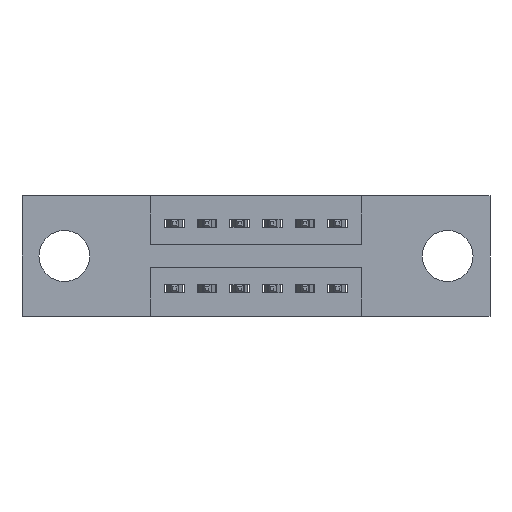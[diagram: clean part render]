
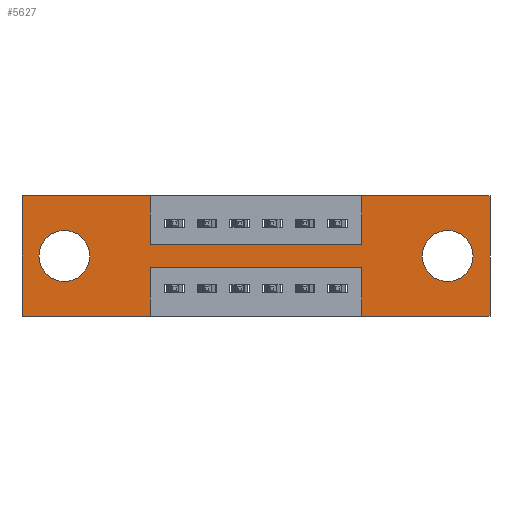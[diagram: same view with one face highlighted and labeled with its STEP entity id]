
A CAD part, front view. The second image highlights one B-rep face of the part: STEP entity #5627.
In plain terms, the highlighted planar face has unit normal (0, -1, 0).
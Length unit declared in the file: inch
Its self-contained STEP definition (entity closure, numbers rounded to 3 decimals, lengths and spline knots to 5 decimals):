
#52 = DIRECTION ( 'NONE',  ( 1., 0., 0. ) ) ;
#59 = DIRECTION ( 'NONE',  ( 0., 0., -1. ) ) ;
#96 = VERTEX_POINT ( 'NONE', #4070 ) ;
#128 = CARTESIAN_POINT ( 'NONE',  ( 0.3925, 0., -0.37 ) ) ;
#204 = DIRECTION ( 'NONE',  ( 0., 0., 1. ) ) ;
#215 = CARTESIAN_POINT ( 'NONE',  ( 0., 0., -0.37 ) ) ;
#245 = VERTEX_POINT ( 'NONE', #5455 ) ;
#251 = CARTESIAN_POINT ( 'NONE',  ( 0.13, 0., -0.263 ) ) ;
#255 = EDGE_CURVE ( 'NONE', #1596, #6113, #8047, .T. ) ;
#288 = VERTEX_POINT ( 'NONE', #5381 ) ;
#326 = DIRECTION ( 'NONE',  ( -1., 0., 0. ) ) ;
#418 = DIRECTION ( 'NONE',  ( 0., 0., -1. ) ) ;
#671 = VECTOR ( 'NONE', #3978, 39.37008 ) ;
#684 = VECTOR ( 'NONE', #4832, 39.37008 ) ;
#730 = EDGE_LOOP ( 'NONE', ( #4895, #5170, #6230, #2188, #3223, #6714, #6895, #7309, #1668, #2954, #6140, #4345 ) ) ;
#1065 = VECTOR ( 'NONE', #418, 39.37008 ) ;
#1235 = CARTESIAN_POINT ( 'NONE',  ( 1.0425, 0., -0.37 ) ) ;
#1316 = AXIS2_PLACEMENT_3D ( 'NONE', #3298, #4785, #3431 ) ;
#1321 = VECTOR ( 'NONE', #9518, 39.37008 ) ;
#1490 = LINE ( 'NONE', #128, #671 ) ;
#1502 = CIRCLE ( 'NONE', #3021, 0.078 ) ;
#1596 = VERTEX_POINT ( 'NONE', #9465 ) ;
#1601 = CARTESIAN_POINT ( 'NONE',  ( 0.13, 0., -0.185 ) ) ;
#1655 = EDGE_CURVE ( 'NONE', #3205, #96, #9492, .T. ) ;
#1668 = ORIENTED_EDGE ( 'NONE', *, *, #4088, .F. ) ;
#1682 = DIRECTION ( 'NONE',  ( -1., 0., 0. ) ) ;
#1746 = VECTOR ( 'NONE', #4020, 39.37008 ) ;
#1764 = CARTESIAN_POINT ( 'NONE',  ( 0., 0., -0.37 ) ) ;
#1768 = CARTESIAN_POINT ( 'NONE',  ( 0.13, 0., -0.107 ) ) ;
#1769 = CARTESIAN_POINT ( 'NONE',  ( 1.0425, 0., -0.37 ) ) ;
#1796 = PLANE ( 'NONE',  #1316 ) ;
#1809 = EDGE_CURVE ( 'NONE', #96, #3949, #3054, .T. ) ;
#1904 = VERTEX_POINT ( 'NONE', #7506 ) ;
#1940 = VERTEX_POINT ( 'NONE', #1768 ) ;
#1958 = VERTEX_POINT ( 'NONE', #5801 ) ;
#1961 = EDGE_CURVE ( 'NONE', #1904, #245, #5511, .T. ) ;
#2014 = AXIS2_PLACEMENT_3D ( 'NONE', #1601, #6901, #6769 ) ;
#2158 = VECTOR ( 'NONE', #9476, 39.37008 ) ;
#2188 = ORIENTED_EDGE ( 'NONE', *, *, #1809, .F. ) ;
#2269 = CARTESIAN_POINT ( 'NONE',  ( 0., 0., -0.37 ) ) ;
#2553 = CARTESIAN_POINT ( 'NONE',  ( 0., 0., 0. ) ) ;
#2802 = EDGE_LOOP ( 'NONE', ( #7205, #4840 ) ) ;
#2829 = EDGE_CURVE ( 'NONE', #3949, #3636, #3279, .T. ) ;
#2834 = VECTOR ( 'NONE', #1682, 39.37008 ) ;
#2954 = ORIENTED_EDGE ( 'NONE', *, *, #9488, .F. ) ;
#3003 = CIRCLE ( 'NONE', #2014, 0.078 ) ;
#3021 = AXIS2_PLACEMENT_3D ( 'NONE', #6451, #8053, #9486 ) ;
#3054 = LINE ( 'NONE', #215, #2834 ) ;
#3205 = VERTEX_POINT ( 'NONE', #8108 ) ;
#3223 = ORIENTED_EDGE ( 'NONE', *, *, #1655, .F. ) ;
#3234 = VECTOR ( 'NONE', #52, 39.37008 ) ;
#3279 = LINE ( 'NONE', #1235, #4992 ) ;
#3298 = CARTESIAN_POINT ( 'NONE',  ( 0., 0., -0.37 ) ) ;
#3431 = DIRECTION ( 'NONE',  ( 0., 0., -1. ) ) ;
#3442 = VECTOR ( 'NONE', #326, 39.37008 ) ;
#3522 = AXIS2_PLACEMENT_3D ( 'NONE', #4591, #7476, #59 ) ;
#3636 = VERTEX_POINT ( 'NONE', #5049 ) ;
#3670 = EDGE_CURVE ( 'NONE', #288, #1958, #1502, .T. ) ;
#3869 = AXIS2_PLACEMENT_3D ( 'NONE', #8326, #6138, #204 ) ;
#3942 = DIRECTION ( 'NONE',  ( -1., 0., 0. ) ) ;
#3949 = VERTEX_POINT ( 'NONE', #1769 ) ;
#3978 = DIRECTION ( 'NONE',  ( 0., 0., -1. ) ) ;
#4020 = DIRECTION ( 'NONE',  ( 1., 0., 0. ) ) ;
#4070 = CARTESIAN_POINT ( 'NONE',  ( 1.435, 0., -0.37 ) ) ;
#4077 = CARTESIAN_POINT ( 'NONE',  ( 0.3925, 0., 0. ) ) ;
#4088 = EDGE_CURVE ( 'NONE', #9033, #9016, #5678, .T. ) ;
#4111 = LINE ( 'NONE', #4365, #2158 ) ;
#4345 = ORIENTED_EDGE ( 'NONE', *, *, #255, .F. ) ;
#4365 = CARTESIAN_POINT ( 'NONE',  ( 0.3925, 0., -0.15 ) ) ;
#4591 = CARTESIAN_POINT ( 'NONE',  ( 1.305, 0., -0.185 ) ) ;
#4596 = EDGE_CURVE ( 'NONE', #245, #3205, #8671, .T. ) ;
#4785 = DIRECTION ( 'NONE',  ( 0., -1., 0. ) ) ;
#4832 = DIRECTION ( 'NONE',  ( 0., 0., -1. ) ) ;
#4840 = ORIENTED_EDGE ( 'NONE', *, *, #7599, .T. ) ;
#4895 = ORIENTED_EDGE ( 'NONE', *, *, #8859, .F. ) ;
#4992 = VECTOR ( 'NONE', #6426, 39.37008 ) ;
#5049 = CARTESIAN_POINT ( 'NONE',  ( 1.0425, 0., -0.22 ) ) ;
#5170 = ORIENTED_EDGE ( 'NONE', *, *, #6563, .F. ) ;
#5381 = CARTESIAN_POINT ( 'NONE',  ( 1.305, 0., -0.107 ) ) ;
#5455 = CARTESIAN_POINT ( 'NONE',  ( 1.0425, 0., 0. ) ) ;
#5511 = LINE ( 'NONE', #5829, #1321 ) ;
#5627 = ADVANCED_FACE ( 'NONE', ( #7832, #8531, #5889 ), #1796, .T. ) ;
#5678 = LINE ( 'NONE', #4077, #684 ) ;
#5742 = CIRCLE ( 'NONE', #3869, 0.078 ) ;
#5787 = ORIENTED_EDGE ( 'NONE', *, *, #5802, .T. ) ;
#5801 = CARTESIAN_POINT ( 'NONE',  ( 1.305, 0., -0.263 ) ) ;
#5802 = EDGE_CURVE ( 'NONE', #8919, #1940, #3003, .T. ) ;
#5829 = CARTESIAN_POINT ( 'NONE',  ( 1.0425, 0., 0. ) ) ;
#5866 = VERTEX_POINT ( 'NONE', #6833 ) ;
#5889 = FACE_OUTER_BOUND ( 'NONE', #730, .T. ) ;
#5911 = CARTESIAN_POINT ( 'NONE',  ( 0., 0., 0. ) ) ;
#6113 = VERTEX_POINT ( 'NONE', #2269 ) ;
#6138 = DIRECTION ( 'NONE',  ( 0., 1., 0. ) ) ;
#6140 = ORIENTED_EDGE ( 'NONE', *, *, #9385, .F. ) ;
#6230 = ORIENTED_EDGE ( 'NONE', *, *, #2829, .F. ) ;
#6348 = CARTESIAN_POINT ( 'NONE',  ( 0.3925, 0., 0. ) ) ;
#6375 = CARTESIAN_POINT ( 'NONE',  ( 0.3925, 0., -0.15 ) ) ;
#6389 = CARTESIAN_POINT ( 'NONE',  ( 1.435, 0., 0. ) ) ;
#6417 = VERTEX_POINT ( 'NONE', #6767 ) ;
#6426 = DIRECTION ( 'NONE',  ( 0., 0., 1. ) ) ;
#6451 = CARTESIAN_POINT ( 'NONE',  ( 1.305, 0., -0.185 ) ) ;
#6563 = EDGE_CURVE ( 'NONE', #3636, #5866, #8282, .T. ) ;
#6664 = CIRCLE ( 'NONE', #3522, 0.078 ) ;
#6714 = ORIENTED_EDGE ( 'NONE', *, *, #4596, .F. ) ;
#6767 = CARTESIAN_POINT ( 'NONE',  ( 0., 0., 0. ) ) ;
#6769 = DIRECTION ( 'NONE',  ( 0., 0., 1. ) ) ;
#6796 = EDGE_CURVE ( 'NONE', #9016, #1904, #4111, .T. ) ;
#6833 = CARTESIAN_POINT ( 'NONE',  ( 0.3925, 0., -0.22 ) ) ;
#6895 = ORIENTED_EDGE ( 'NONE', *, *, #1961, .F. ) ;
#6901 = DIRECTION ( 'NONE',  ( 0., 1., 0. ) ) ;
#7057 = VECTOR ( 'NONE', #7663, 39.37008 ) ;
#7133 = VECTOR ( 'NONE', #3942, 39.37008 ) ;
#7205 = ORIENTED_EDGE ( 'NONE', *, *, #3670, .T. ) ;
#7309 = ORIENTED_EDGE ( 'NONE', *, *, #6796, .F. ) ;
#7361 = EDGE_CURVE ( 'NONE', #1940, #8919, #5742, .T. ) ;
#7476 = DIRECTION ( 'NONE',  ( 0., 1., 0. ) ) ;
#7506 = CARTESIAN_POINT ( 'NONE',  ( 1.0425, 0., -0.15 ) ) ;
#7530 = ORIENTED_EDGE ( 'NONE', *, *, #7361, .T. ) ;
#7599 = EDGE_CURVE ( 'NONE', #1958, #288, #6664, .T. ) ;
#7663 = DIRECTION ( 'NONE',  ( 0., 0., 1. ) ) ;
#7721 = LINE ( 'NONE', #5911, #3234 ) ;
#7817 = EDGE_LOOP ( 'NONE', ( #7530, #5787 ) ) ;
#7832 = FACE_BOUND ( 'NONE', #2802, .T. ) ;
#7972 = LINE ( 'NONE', #2553, #7057 ) ;
#8047 = LINE ( 'NONE', #1764, #3442 ) ;
#8053 = DIRECTION ( 'NONE',  ( 0., 1., 0. ) ) ;
#8108 = CARTESIAN_POINT ( 'NONE',  ( 1.435, 0., 0. ) ) ;
#8282 = LINE ( 'NONE', #8426, #7133 ) ;
#8326 = CARTESIAN_POINT ( 'NONE',  ( 0.13, 0., -0.185 ) ) ;
#8426 = CARTESIAN_POINT ( 'NONE',  ( 0.3925, 0., -0.22 ) ) ;
#8442 = CARTESIAN_POINT ( 'NONE',  ( 0., 0., 0. ) ) ;
#8531 = FACE_BOUND ( 'NONE', #7817, .T. ) ;
#8671 = LINE ( 'NONE', #8442, #1746 ) ;
#8859 = EDGE_CURVE ( 'NONE', #5866, #1596, #1490, .T. ) ;
#8919 = VERTEX_POINT ( 'NONE', #251 ) ;
#9016 = VERTEX_POINT ( 'NONE', #6375 ) ;
#9033 = VERTEX_POINT ( 'NONE', #6348 ) ;
#9385 = EDGE_CURVE ( 'NONE', #6113, #6417, #7972, .T. ) ;
#9465 = CARTESIAN_POINT ( 'NONE',  ( 0.3925, 0., -0.37 ) ) ;
#9476 = DIRECTION ( 'NONE',  ( 1., 0., 0. ) ) ;
#9486 = DIRECTION ( 'NONE',  ( 0., 0., -1. ) ) ;
#9488 = EDGE_CURVE ( 'NONE', #6417, #9033, #7721, .T. ) ;
#9492 = LINE ( 'NONE', #6389, #1065 ) ;
#9518 = DIRECTION ( 'NONE',  ( 0., 0., 1. ) ) ;
